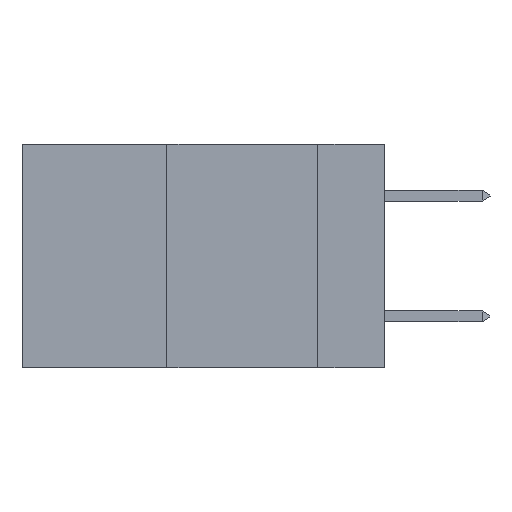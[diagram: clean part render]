
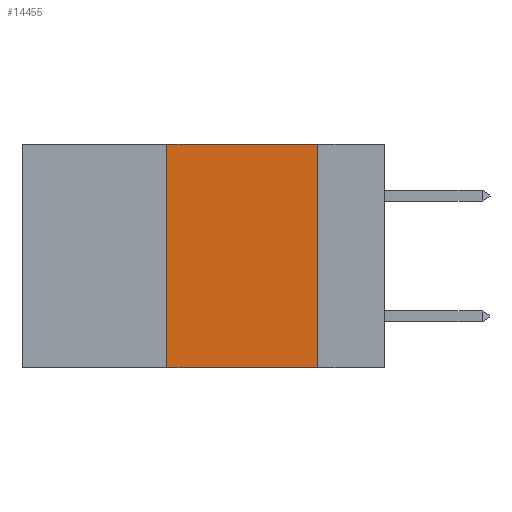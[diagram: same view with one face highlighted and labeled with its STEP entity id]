
A CAD part, left-side view. The second image highlights one B-rep face of the part: STEP entity #14455.
In plain terms, the highlighted planar face has unit normal (-1, 0, 0).
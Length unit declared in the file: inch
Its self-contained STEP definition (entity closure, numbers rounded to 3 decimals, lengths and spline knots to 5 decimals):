
#435 = FACE_OUTER_BOUND ( 'NONE', #16166, .T. ) ;
#1420 = CARTESIAN_POINT ( 'NONE',  ( 0., 0.36, 0. ) ) ;
#2180 = ORIENTED_EDGE ( 'NONE', *, *, #14905, .T. ) ;
#2334 = LINE ( 'NONE', #12858, #17234 ) ;
#3173 = ORIENTED_EDGE ( 'NONE', *, *, #9057, .F. ) ;
#5043 = DIRECTION ( 'NONE',  ( 0., 0., -1. ) ) ;
#5181 = CARTESIAN_POINT ( 'NONE',  ( 0., 0.6, 0. ) ) ;
#6962 = EDGE_CURVE ( 'NONE', #21600, #26156, #2334, .T. ) ;
#9057 = EDGE_CURVE ( 'NONE', #12592, #9712, #10627, .T. ) ;
#9120 = CARTESIAN_POINT ( 'NONE',  ( 0., 0.11, -0.37 ) ) ;
#9712 = VERTEX_POINT ( 'NONE', #26441 ) ;
#10047 = DIRECTION ( 'NONE',  ( 0., 0., 1. ) ) ;
#10627 = LINE ( 'NONE', #1420, #16029 ) ;
#11073 = EDGE_CURVE ( 'NONE', #9712, #21600, #27161, .T. ) ;
#11678 = ORIENTED_EDGE ( 'NONE', *, *, #6962, .F. ) ;
#11684 = VECTOR ( 'NONE', #20532, 39.37008 ) ;
#11688 = CARTESIAN_POINT ( 'NONE',  ( 0., 0.36, -0.37 ) ) ;
#12023 = CARTESIAN_POINT ( 'NONE',  ( 0., 0.6, -0.37 ) ) ;
#12592 = VERTEX_POINT ( 'NONE', #11688 ) ;
#12858 = CARTESIAN_POINT ( 'NONE',  ( 0., 0.11, 0. ) ) ;
#13890 = ORIENTED_EDGE ( 'NONE', *, *, #11073, .F. ) ;
#14100 = DIRECTION ( 'NONE',  ( 1., 0., 0. ) ) ;
#14455 = ADVANCED_FACE ( 'NONE', ( #435 ), #15966, .F. ) ;
#14905 = EDGE_CURVE ( 'NONE', #12592, #26156, #25254, .T. ) ;
#15102 = CARTESIAN_POINT ( 'NONE',  ( 0., 0.11, 0. ) ) ;
#15966 = PLANE ( 'NONE',  #28220 ) ;
#16029 = VECTOR ( 'NONE', #10047, 39.37008 ) ;
#16166 = EDGE_LOOP ( 'NONE', ( #11678, #13890, #3173, #2180 ) ) ;
#17234 = VECTOR ( 'NONE', #17305, 39.37008 ) ;
#17305 = DIRECTION ( 'NONE',  ( 0., 0., -1. ) ) ;
#18068 = DIRECTION ( 'NONE',  ( 0., -1., 0. ) ) ;
#18493 = VECTOR ( 'NONE', #18068, 39.37008 ) ;
#20532 = DIRECTION ( 'NONE',  ( 0., -1., 0. ) ) ;
#21600 = VERTEX_POINT ( 'NONE', #15102 ) ;
#24838 = CARTESIAN_POINT ( 'NONE',  ( 0., 0.6, 0. ) ) ;
#25254 = LINE ( 'NONE', #12023, #11684 ) ;
#26156 = VERTEX_POINT ( 'NONE', #9120 ) ;
#26441 = CARTESIAN_POINT ( 'NONE',  ( 0., 0.36, 0. ) ) ;
#27161 = LINE ( 'NONE', #24838, #18493 ) ;
#28220 = AXIS2_PLACEMENT_3D ( 'NONE', #5181, #14100, #5043 ) ;
